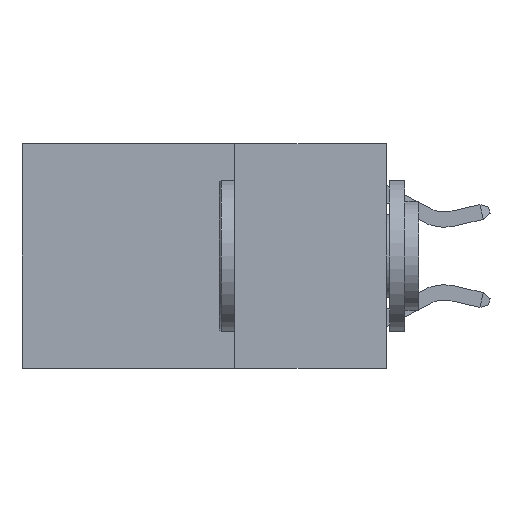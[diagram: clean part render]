
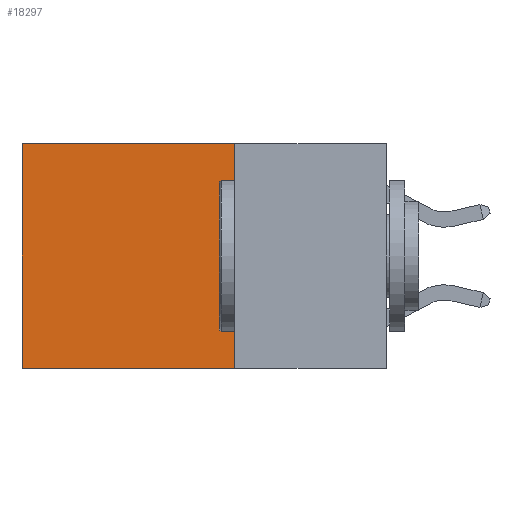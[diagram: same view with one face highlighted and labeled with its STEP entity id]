
A CAD part, left-side view. The second image highlights one B-rep face of the part: STEP entity #18297.
In plain terms, the highlighted planar face has unit normal (-1, 0, 0).
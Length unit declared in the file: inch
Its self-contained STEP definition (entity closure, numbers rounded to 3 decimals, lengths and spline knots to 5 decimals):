
#1050 = CARTESIAN_POINT ( 'NONE',  ( 0.2625, 0.6, -0.37 ) ) ;
#1089 = EDGE_LOOP ( 'NONE', ( #19822, #23324, #18584, #13415 ) ) ;
#1153 = EDGE_CURVE ( 'NONE', #1352, #13220, #14873, .T. ) ;
#1352 = VERTEX_POINT ( 'NONE', #6719 ) ;
#1551 = CARTESIAN_POINT ( 'NONE',  ( 0.2625, 0.25, -0.37 ) ) ;
#1772 = PLANE ( 'NONE',  #9668 ) ;
#1899 = FACE_OUTER_BOUND ( 'NONE', #1089, .T. ) ;
#4205 = CARTESIAN_POINT ( 'NONE',  ( 0.2625, 0.6, 0. ) ) ;
#5193 = VERTEX_POINT ( 'NONE', #1050 ) ;
#6160 = EDGE_CURVE ( 'NONE', #13220, #5193, #7417, .T. ) ;
#6719 = CARTESIAN_POINT ( 'NONE',  ( 0.2625, 0.25, 0. ) ) ;
#7239 = VECTOR ( 'NONE', #10230, 39.37008 ) ;
#7417 = LINE ( 'NONE', #22057, #16316 ) ;
#7984 = EDGE_CURVE ( 'NONE', #1352, #23200, #19386, .T. ) ;
#9668 = AXIS2_PLACEMENT_3D ( 'NONE', #21686, #16211, #23461 ) ;
#10230 = DIRECTION ( 'NONE',  ( 0., 0., -1. ) ) ;
#11286 = CARTESIAN_POINT ( 'NONE',  ( 0.2625, 0.25, 0. ) ) ;
#12005 = CARTESIAN_POINT ( 'NONE',  ( 0.2625, 0.25, 0. ) ) ;
#12896 = DIRECTION ( 'NONE',  ( 0., 0., -1. ) ) ;
#13065 = DIRECTION ( 'NONE',  ( 0., 1., 0. ) ) ;
#13220 = VERTEX_POINT ( 'NONE', #4205 ) ;
#13415 = ORIENTED_EDGE ( 'NONE', *, *, #1153, .T. ) ;
#14873 = LINE ( 'NONE', #11286, #22263 ) ;
#16211 = DIRECTION ( 'NONE',  ( 1., 0., 0. ) ) ;
#16316 = VECTOR ( 'NONE', #12896, 39.37008 ) ;
#16411 = EDGE_CURVE ( 'NONE', #23200, #5193, #19669, .T. ) ;
#17657 = DIRECTION ( 'NONE',  ( 0., 1., 0. ) ) ;
#18203 = VECTOR ( 'NONE', #17657, 39.37008 ) ;
#18297 = ADVANCED_FACE ( 'NONE', ( #1899 ), #1772, .F. ) ;
#18584 = ORIENTED_EDGE ( 'NONE', *, *, #7984, .F. ) ;
#19386 = LINE ( 'NONE', #12005, #7239 ) ;
#19669 = LINE ( 'NONE', #1551, #18203 ) ;
#19822 = ORIENTED_EDGE ( 'NONE', *, *, #6160, .T. ) ;
#20116 = CARTESIAN_POINT ( 'NONE',  ( 0.2625, 0.25, -0.37 ) ) ;
#21686 = CARTESIAN_POINT ( 'NONE',  ( 0.2625, 0.25, 0. ) ) ;
#22057 = CARTESIAN_POINT ( 'NONE',  ( 0.2625, 0.6, 0. ) ) ;
#22263 = VECTOR ( 'NONE', #13065, 39.37008 ) ;
#23200 = VERTEX_POINT ( 'NONE', #20116 ) ;
#23324 = ORIENTED_EDGE ( 'NONE', *, *, #16411, .F. ) ;
#23461 = DIRECTION ( 'NONE',  ( 0., 0., -1. ) ) ;
